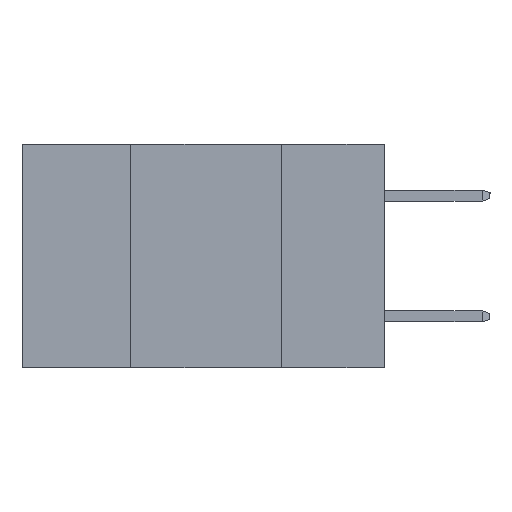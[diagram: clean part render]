
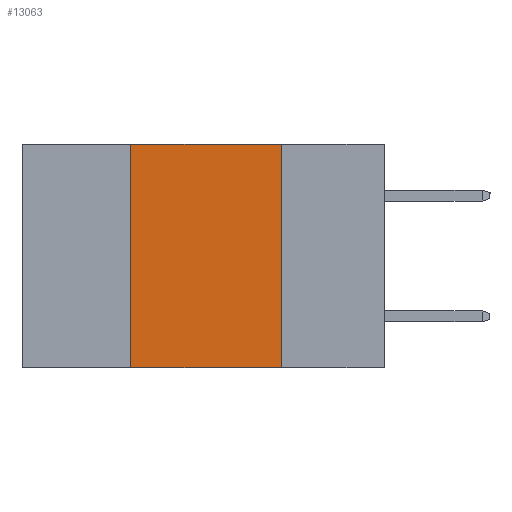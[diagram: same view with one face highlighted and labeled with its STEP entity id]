
A CAD part, left-side view. The second image highlights one B-rep face of the part: STEP entity #13063.
In plain terms, the highlighted planar face has unit normal (-1, 0, 0).
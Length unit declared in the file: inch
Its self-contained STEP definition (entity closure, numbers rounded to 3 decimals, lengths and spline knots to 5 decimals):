
#344 = EDGE_CURVE ( 'NONE', #8721, #4154, #4564, .T. ) ;
#2091 = VECTOR ( 'NONE', #2827, 39.37008 ) ;
#2101 = LINE ( 'NONE', #6242, #8641 ) ;
#2308 = CARTESIAN_POINT ( 'NONE',  ( 0., 0.6, 0. ) ) ;
#2631 = CARTESIAN_POINT ( 'NONE',  ( 0., 0.17, -0.37 ) ) ;
#2740 = DIRECTION ( 'NONE',  ( 0., 0., 1. ) ) ;
#2827 = DIRECTION ( 'NONE',  ( 0., -1., 0. ) ) ;
#2960 = CARTESIAN_POINT ( 'NONE',  ( 0., 0.17, 0. ) ) ;
#3039 = CARTESIAN_POINT ( 'NONE',  ( 0., 0.42, 0. ) ) ;
#4154 = VERTEX_POINT ( 'NONE', #3039 ) ;
#4564 = LINE ( 'NONE', #6863, #9973 ) ;
#4654 = LINE ( 'NONE', #2631, #5035 ) ;
#4845 = CARTESIAN_POINT ( 'NONE',  ( 0., 0.6, -0.37 ) ) ;
#5035 = VECTOR ( 'NONE', #5883, 39.37008 ) ;
#5413 = ORIENTED_EDGE ( 'NONE', *, *, #344, .F. ) ;
#5618 = ORIENTED_EDGE ( 'NONE', *, *, #5774, .F. ) ;
#5774 = EDGE_CURVE ( 'NONE', #7328, #12564, #4654, .T. ) ;
#5819 = AXIS2_PLACEMENT_3D ( 'NONE', #2308, #6250, #6315 ) ;
#5883 = DIRECTION ( 'NONE',  ( 0., 0., -1. ) ) ;
#6033 = CARTESIAN_POINT ( 'NONE',  ( 0., 0.42, -0.37 ) ) ;
#6236 = ORIENTED_EDGE ( 'NONE', *, *, #9231, .T. ) ;
#6242 = CARTESIAN_POINT ( 'NONE',  ( 0., 0.6, 0. ) ) ;
#6250 = DIRECTION ( 'NONE',  ( 1., 0., 0. ) ) ;
#6315 = DIRECTION ( 'NONE',  ( 0., 0., -1. ) ) ;
#6527 = CARTESIAN_POINT ( 'NONE',  ( 0., 0.17, -0.37 ) ) ;
#6863 = CARTESIAN_POINT ( 'NONE',  ( 0., 0.42, -0.37 ) ) ;
#7325 = FACE_OUTER_BOUND ( 'NONE', #13177, .T. ) ;
#7328 = VERTEX_POINT ( 'NONE', #2960 ) ;
#8641 = VECTOR ( 'NONE', #10385, 39.37008 ) ;
#8721 = VERTEX_POINT ( 'NONE', #6033 ) ;
#9231 = EDGE_CURVE ( 'NONE', #8721, #12564, #10084, .T. ) ;
#9973 = VECTOR ( 'NONE', #2740, 39.37008 ) ;
#10084 = LINE ( 'NONE', #4845, #2091 ) ;
#10385 = DIRECTION ( 'NONE',  ( 0., -1., 0. ) ) ;
#11515 = EDGE_CURVE ( 'NONE', #4154, #7328, #2101, .T. ) ;
#11850 = ORIENTED_EDGE ( 'NONE', *, *, #11515, .F. ) ;
#12337 = PLANE ( 'NONE',  #5819 ) ;
#12564 = VERTEX_POINT ( 'NONE', #6527 ) ;
#13063 = ADVANCED_FACE ( 'NONE', ( #7325 ), #12337, .F. ) ;
#13177 = EDGE_LOOP ( 'NONE', ( #5618, #11850, #5413, #6236 ) ) ;
